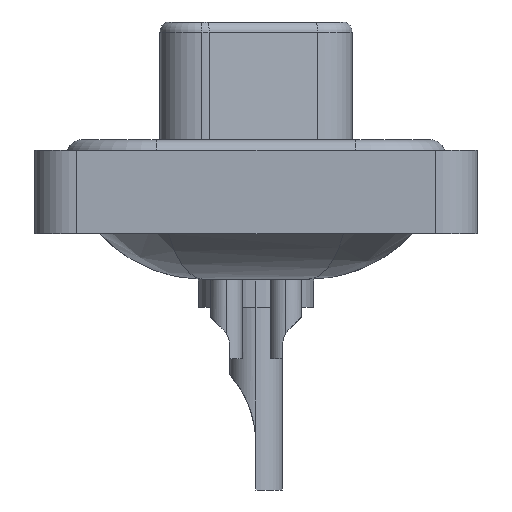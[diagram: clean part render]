
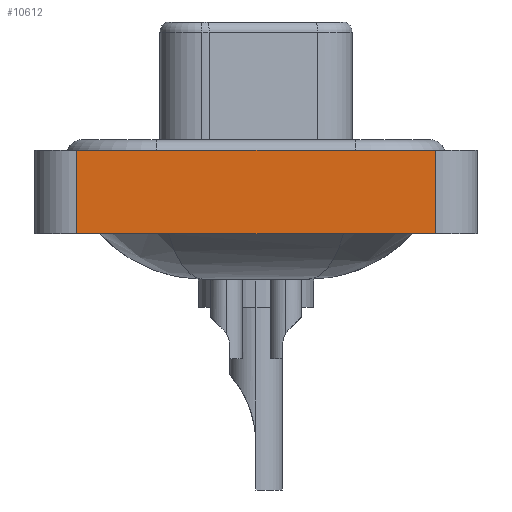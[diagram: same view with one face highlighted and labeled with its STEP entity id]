
A CAD part, left-side view. The second image highlights one B-rep face of the part: STEP entity #10612.
In plain terms, the highlighted planar face has unit normal (-1, 0, 0).
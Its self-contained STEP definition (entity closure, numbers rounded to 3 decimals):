
#349 = DIRECTION ( 'NONE',  ( -1., 0., 0. ) ) ;
#1092 = EDGE_LOOP ( 'NONE', ( #3738, #17308, #13286, #15617 ) ) ;
#1591 = LINE ( 'NONE', #14140, #1672 ) ;
#1672 = VECTOR ( 'NONE', #5834, 1000. ) ;
#2628 = EDGE_CURVE ( 'NONE', #4622, #3657, #5927, .T. ) ;
#2644 = LINE ( 'NONE', #13750, #13439 ) ;
#3230 = VERTEX_POINT ( 'NONE', #4720 ) ;
#3657 = VERTEX_POINT ( 'NONE', #8852 ) ;
#3738 = ORIENTED_EDGE ( 'NONE', *, *, #11094, .T. ) ;
#4622 = VERTEX_POINT ( 'NONE', #12459 ) ;
#4680 = CARTESIAN_POINT ( 'NONE',  ( -7.25, -8.55, -3.6 ) ) ;
#4720 = CARTESIAN_POINT ( 'NONE',  ( -7.25, -8.55, -3.6 ) ) ;
#5623 = DIRECTION ( 'NONE',  ( 0., -1., 0. ) ) ;
#5748 = CARTESIAN_POINT ( 'NONE',  ( -7.25, 8.55, -3.6 ) ) ;
#5834 = DIRECTION ( 'NONE',  ( 0., 0., 1. ) ) ;
#5927 = LINE ( 'NONE', #5748, #14063 ) ;
#7089 = CARTESIAN_POINT ( 'NONE',  ( -7.25, -8.55, 0.4 ) ) ;
#7169 = CARTESIAN_POINT ( 'NONE',  ( -7.25, -8.55, 0.4 ) ) ;
#7676 = VECTOR ( 'NONE', #14044, 1000. ) ;
#8852 = CARTESIAN_POINT ( 'NONE',  ( -7.25, 8.55, 0.4 ) ) ;
#10016 = PLANE ( 'NONE',  #13356 ) ;
#10612 = ADVANCED_FACE ( 'NONE', ( #17061 ), #10016, .T. ) ;
#11094 = EDGE_CURVE ( 'NONE', #3230, #16314, #1591, .T. ) ;
#12459 = CARTESIAN_POINT ( 'NONE',  ( -7.25, 8.55, -3.6 ) ) ;
#12688 = DIRECTION ( 'NONE',  ( 0., 0., 1. ) ) ;
#12848 = EDGE_CURVE ( 'NONE', #3657, #16314, #15660, .T. ) ;
#12991 = DIRECTION ( 'NONE',  ( 0., 0., 1. ) ) ;
#13286 = ORIENTED_EDGE ( 'NONE', *, *, #2628, .F. ) ;
#13356 = AXIS2_PLACEMENT_3D ( 'NONE', #4680, #349, #12991 ) ;
#13439 = VECTOR ( 'NONE', #5623, 1000. ) ;
#13750 = CARTESIAN_POINT ( 'NONE',  ( -7.25, -8.55, -3.6 ) ) ;
#14044 = DIRECTION ( 'NONE',  ( 0., -1., 0. ) ) ;
#14063 = VECTOR ( 'NONE', #12688, 1000. ) ;
#14140 = CARTESIAN_POINT ( 'NONE',  ( -7.25, -8.55, -3.6 ) ) ;
#14748 = EDGE_CURVE ( 'NONE', #4622, #3230, #2644, .T. ) ;
#15617 = ORIENTED_EDGE ( 'NONE', *, *, #14748, .T. ) ;
#15660 = LINE ( 'NONE', #7089, #7676 ) ;
#16314 = VERTEX_POINT ( 'NONE', #7169 ) ;
#17061 = FACE_OUTER_BOUND ( 'NONE', #1092, .T. ) ;
#17308 = ORIENTED_EDGE ( 'NONE', *, *, #12848, .F. ) ;
